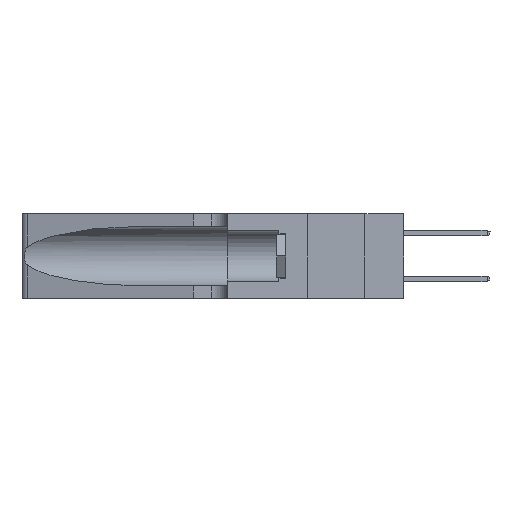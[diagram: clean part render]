
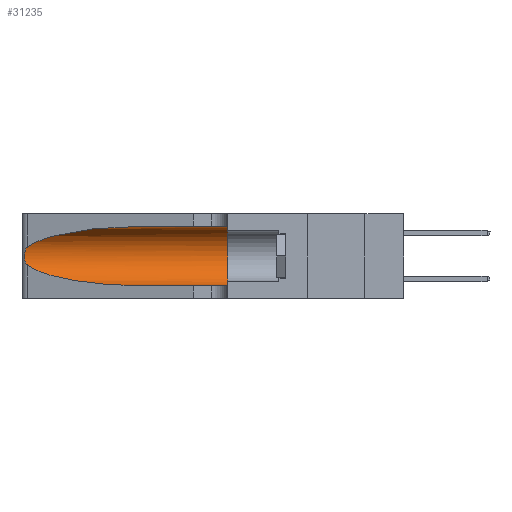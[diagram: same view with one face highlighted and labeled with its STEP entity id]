
A CAD part, left-side view. The second image highlights one B-rep face of the part: STEP entity #31235.
In plain terms, the highlighted cylindrical face has radius 3.308 mm (diameter 6.617 mm), a partial arc.
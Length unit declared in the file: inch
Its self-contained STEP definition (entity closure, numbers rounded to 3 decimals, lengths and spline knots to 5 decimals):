
#586 = CARTESIAN_POINT ( 'NONE',  ( 0.25487, 1.22718, 0.22369 ) ) ;
#896 = DIRECTION ( 'NONE',  ( 0., -1., 0. ) ) ;
#2055 = CARTESIAN_POINT ( 'NONE',  ( 0.25639, 1.23184, 0.21858 ) ) ;
#2062 = CYLINDRICAL_SURFACE ( 'NONE', #4018, 0.13025 ) ;
#2210 = CARTESIAN_POINT ( 'NONE',  ( 0.25487, 1.22718, 0.14631 ) ) ;
#3846 = VECTOR ( 'NONE', #36070, 39.37008 ) ;
#4018 = AXIS2_PLACEMENT_3D ( 'NONE', #4515, #896, #25450 ) ;
#4515 = CARTESIAN_POINT ( 'NONE',  ( 0.1305, 1.61858, 0.185 ) ) ;
#6825 = VERTEX_POINT ( 'NONE', #38551 ) ;
#8317 = CARTESIAN_POINT ( 'NONE',  ( 0.1305, 0.72297, 0.05475 ) ) ;
#9187 = CARTESIAN_POINT ( 'NONE',  ( 0.25854, 1.2359, 0.20912 ) ) ;
#10369 = EDGE_CURVE ( 'NONE', #34637, #28041, #21917, .T. ) ;
#10757 = EDGE_CURVE ( 'NONE', #15485, #34637, #13778, .T. ) ;
#11386 = CARTESIAN_POINT ( 'NONE',  ( 0.18966, 0.96281, 0.05475 ) ) ;
#12583 = FACE_OUTER_BOUND ( 'NONE', #16741, .T. ) ;
#12724 = CARTESIAN_POINT ( 'NONE',  ( 0.26075, 1.23896, 0.19203 ) ) ;
#13378 = CARTESIAN_POINT ( 'NONE',  ( 0.1305, 0.72297, 0.31525 ) ) ;
#13778 =( BOUNDED_CURVE ( )  B_SPLINE_CURVE ( 3, ( #14669, #18213, #21712, #586 ),
 .UNSPECIFIED., .F., .T. ) 
 B_SPLINE_CURVE_WITH_KNOTS ( ( 4, 4 ),
 ( 1.5708, 2.84003 ),
 .UNSPECIFIED. ) 
 CURVE ( )  GEOMETRIC_REPRESENTATION_ITEM ( )  RATIONAL_B_SPLINE_CURVE ( ( 1., 0.87, 0.87, 1. ) ) 
 REPRESENTATION_ITEM ( '' )  );
#14002 = CIRCLE ( 'NONE', #36845, 0.13025 ) ;
#14033 = CARTESIAN_POINT ( 'NONE',  ( 0.25487, 1.22718, 0.22369 ) ) ;
#14669 = CARTESIAN_POINT ( 'NONE',  ( 0.1305, 0.72297, 0.31525 ) ) ;
#15155 = VECTOR ( 'NONE', #44059, 39.37008 ) ;
#15409 = CARTESIAN_POINT ( 'NONE',  ( 0.1305, 1.61858, 0.31525 ) ) ;
#15441 = LINE ( 'NONE', #15409, #3846 ) ;
#15485 = VERTEX_POINT ( 'NONE', #13378 ) ;
#15663 = ORIENTED_EDGE ( 'NONE', *, *, #10369, .T. ) ;
#16011 = ORIENTED_EDGE ( 'NONE', *, *, #41177, .T. ) ;
#16267 = CARTESIAN_POINT ( 'NONE',  ( 0.26017, 1.23833, 0.17102 ) ) ;
#16741 = EDGE_LOOP ( 'NONE', ( #32220, #15663, #30351, #16011, #18159, #30687 ) ) ;
#16986 = CARTESIAN_POINT ( 'NONE',  ( 0.1305, 0.35, 0.185 ) ) ;
#17154 = VERTEX_POINT ( 'NONE', #8317 ) ;
#18159 = ORIENTED_EDGE ( 'NONE', *, *, #27702, .F. ) ;
#18213 = CARTESIAN_POINT ( 'NONE',  ( 0.18966, 0.96281, 0.31525 ) ) ;
#19635 = CARTESIAN_POINT ( 'NONE',  ( 0.25555, 1.22994, 0.2215 ) ) ;
#19786 = CARTESIAN_POINT ( 'NONE',  ( 0.25789, 1.23486, 0.15765 ) ) ;
#20507 = DIRECTION ( 'NONE',  ( 0., 0., 1. ) ) ;
#21712 = CARTESIAN_POINT ( 'NONE',  ( 0.2373, 1.15595, 0.28018 ) ) ;
#21917 = B_SPLINE_CURVE_WITH_KNOTS ( 'NONE', 3,
 ( #26546, #19635, #2055, #30007, #9187, #33474, #12724, #36911, #16267, #40379, #19786, #43809, #23250, #2210 ),
 .UNSPECIFIED., .F., .F.,
 ( 4, 2, 2, 2, 2, 2, 4 ),
 ( 0., 0.00027, 0.00053, 0.00107, 0.0016, 0.00187, 0.00214 ),
 .UNSPECIFIED. ) ;
#23250 = CARTESIAN_POINT ( 'NONE',  ( 0.25555, 1.22993, 0.14849 ) ) ;
#23291 =( BOUNDED_CURVE ( )  B_SPLINE_CURVE ( 3, ( #28696, #32014, #11386, #35575 ),
 .UNSPECIFIED., .F., .F. ) 
 B_SPLINE_CURVE_WITH_KNOTS ( ( 4, 4 ),
 ( 3.44316, 4.71239 ),
 .UNSPECIFIED. ) 
 CURVE ( )  GEOMETRIC_REPRESENTATION_ITEM ( )  RATIONAL_B_SPLINE_CURVE ( ( 1., 0.87, 0.87, 1. ) ) 
 REPRESENTATION_ITEM ( '' )  );
#25450 = DIRECTION ( 'NONE',  ( 0., 0., -1. ) ) ;
#26546 = CARTESIAN_POINT ( 'NONE',  ( 0.25487, 1.22718, 0.22369 ) ) ;
#27702 = EDGE_CURVE ( 'NONE', #33777, #6825, #14002, .T. ) ;
#28041 = VERTEX_POINT ( 'NONE', #32512 ) ;
#28696 = CARTESIAN_POINT ( 'NONE',  ( 0.25487, 1.22718, 0.14631 ) ) ;
#30007 = CARTESIAN_POINT ( 'NONE',  ( 0.25787, 1.23484, 0.2124 ) ) ;
#30101 = EDGE_CURVE ( 'NONE', #15485, #33777, #15441, .T. ) ;
#30351 = ORIENTED_EDGE ( 'NONE', *, *, #44525, .T. ) ;
#30687 = ORIENTED_EDGE ( 'NONE', *, *, #30101, .F. ) ;
#31235 = ADVANCED_FACE ( 'NONE', ( #12583 ), #2062, .F. ) ;
#32014 = CARTESIAN_POINT ( 'NONE',  ( 0.2373, 1.15595, 0.08982 ) ) ;
#32220 = ORIENTED_EDGE ( 'NONE', *, *, #10757, .T. ) ;
#32512 = CARTESIAN_POINT ( 'NONE',  ( 0.25487, 1.22718, 0.14631 ) ) ;
#33474 = CARTESIAN_POINT ( 'NONE',  ( 0.26018, 1.23835, 0.19895 ) ) ;
#33777 = VERTEX_POINT ( 'NONE', #44114 ) ;
#34637 = VERTEX_POINT ( 'NONE', #14033 ) ;
#35575 = CARTESIAN_POINT ( 'NONE',  ( 0.1305, 0.72297, 0.05475 ) ) ;
#36070 = DIRECTION ( 'NONE',  ( 0., -1., 0. ) ) ;
#36845 = AXIS2_PLACEMENT_3D ( 'NONE', #16986, #41066, #20507 ) ;
#36911 = CARTESIAN_POINT ( 'NONE',  ( 0.26075, 1.23896, 0.178 ) ) ;
#38551 = CARTESIAN_POINT ( 'NONE',  ( 0.1305, 0.35, 0.05475 ) ) ;
#40379 = CARTESIAN_POINT ( 'NONE',  ( 0.25856, 1.23593, 0.16098 ) ) ;
#40627 = CARTESIAN_POINT ( 'NONE',  ( 0.1305, 1.61858, 0.05475 ) ) ;
#41066 = DIRECTION ( 'NONE',  ( 0., 1., 0. ) ) ;
#41177 = EDGE_CURVE ( 'NONE', #17154, #6825, #42665, .T. ) ;
#42665 = LINE ( 'NONE', #40627, #15155 ) ;
#43809 = CARTESIAN_POINT ( 'NONE',  ( 0.25639, 1.23186, 0.15144 ) ) ;
#44059 = DIRECTION ( 'NONE',  ( 0., -1., 0. ) ) ;
#44114 = CARTESIAN_POINT ( 'NONE',  ( 0.1305, 0.35, 0.31525 ) ) ;
#44525 = EDGE_CURVE ( 'NONE', #28041, #17154, #23291, .T. ) ;
